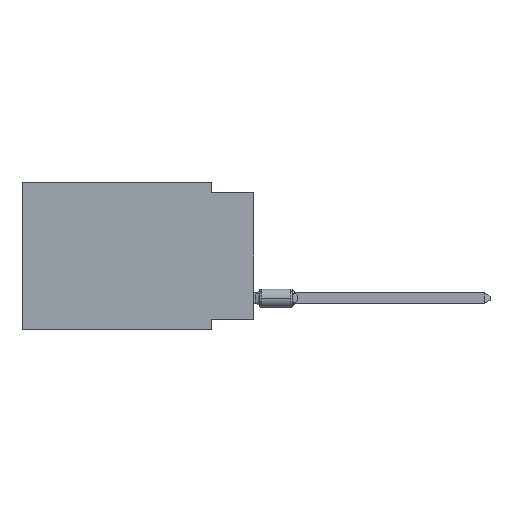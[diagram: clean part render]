
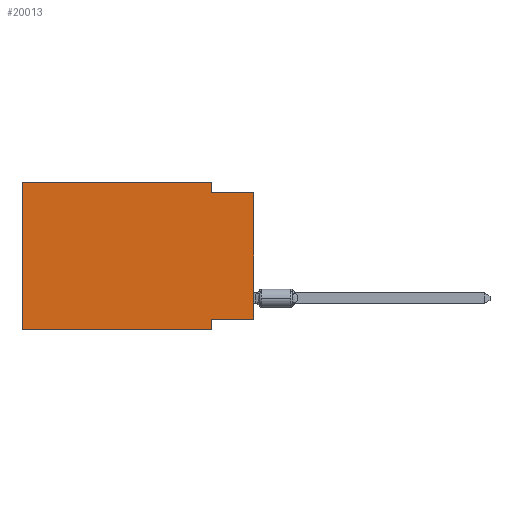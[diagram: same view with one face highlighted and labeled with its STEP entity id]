
A CAD part, left-side view. The second image highlights one B-rep face of the part: STEP entity #20013.
In plain terms, the highlighted planar face has unit normal (-1, 0, 0).
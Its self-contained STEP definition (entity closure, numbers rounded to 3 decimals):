
#96 = CARTESIAN_POINT ( 'NONE',  ( 0., 13.97, -8.89 ) ) ;
#192 = CARTESIAN_POINT ( 'NONE',  ( 0., 2.54, -8.89 ) ) ;
#899 = CARTESIAN_POINT ( 'NONE',  ( 0., 0., 0. ) ) ;
#1477 = DIRECTION ( 'NONE',  ( 0., 0., 1. ) ) ;
#1546 = DIRECTION ( 'NONE',  ( 0., -1., 0. ) ) ;
#1777 = ORIENTED_EDGE ( 'NONE', *, *, #7221, .F. ) ;
#2259 = VERTEX_POINT ( 'NONE', #11842 ) ;
#2874 = VECTOR ( 'NONE', #1546, 1000. ) ;
#2972 = PLANE ( 'NONE',  #17500 ) ;
#3095 = FACE_OUTER_BOUND ( 'NONE', #8683, .T. ) ;
#3350 = CARTESIAN_POINT ( 'NONE',  ( 0., 2.54, -8.255 ) ) ;
#3458 = EDGE_CURVE ( 'NONE', #14503, #10367, #22338, .T. ) ;
#3532 = CARTESIAN_POINT ( 'NONE',  ( 0., 13.97, 0. ) ) ;
#3950 = ORIENTED_EDGE ( 'NONE', *, *, #3458, .F. ) ;
#4339 = DIRECTION ( 'NONE',  ( 0., 0., -1. ) ) ;
#4348 = CARTESIAN_POINT ( 'NONE',  ( 0., 2.54, 0. ) ) ;
#4909 = DIRECTION ( 'NONE',  ( 1., 0., 0. ) ) ;
#5373 = ORIENTED_EDGE ( 'NONE', *, *, #11270, .T. ) ;
#5618 = EDGE_CURVE ( 'NONE', #17515, #2259, #21435, .T. ) ;
#5721 = ORIENTED_EDGE ( 'NONE', *, *, #22646, .F. ) ;
#5803 = CARTESIAN_POINT ( 'NONE',  ( 0., 2.54, 0. ) ) ;
#6016 = VECTOR ( 'NONE', #11324, 1000. ) ;
#6582 = DIRECTION ( 'NONE',  ( 0., 0., 1. ) ) ;
#6608 = VERTEX_POINT ( 'NONE', #96 ) ;
#6885 = VERTEX_POINT ( 'NONE', #3350 ) ;
#7116 = CARTESIAN_POINT ( 'NONE',  ( 0., 0., -0.635 ) ) ;
#7147 = DIRECTION ( 'NONE',  ( 0., -1., 0. ) ) ;
#7221 = EDGE_CURVE ( 'NONE', #6608, #21553, #20195, .T. ) ;
#7418 = CARTESIAN_POINT ( 'NONE',  ( 0., 13.97, -8.89 ) ) ;
#7873 = VECTOR ( 'NONE', #16521, 1000. ) ;
#8683 = EDGE_LOOP ( 'NONE', ( #16354, #18234, #3950, #23668, #1777, #5373, #22352, #5721 ) ) ;
#8732 = CARTESIAN_POINT ( 'NONE',  ( 0., 2.54, -0.635 ) ) ;
#9247 = VERTEX_POINT ( 'NONE', #23162 ) ;
#9518 = VECTOR ( 'NONE', #21668, 1000. ) ;
#10367 = VERTEX_POINT ( 'NONE', #8732 ) ;
#10372 = EDGE_CURVE ( 'NONE', #21553, #14503, #19822, .T. ) ;
#10519 = LINE ( 'NONE', #7116, #2874 ) ;
#10752 = EDGE_CURVE ( 'NONE', #10367, #2259, #10519, .T. ) ;
#11270 = EDGE_CURVE ( 'NONE', #6608, #9247, #12736, .T. ) ;
#11324 = DIRECTION ( 'NONE',  ( 0., 1., 0. ) ) ;
#11842 = CARTESIAN_POINT ( 'NONE',  ( 0., 0., -0.635 ) ) ;
#12736 = LINE ( 'NONE', #7418, #9518 ) ;
#13602 = CARTESIAN_POINT ( 'NONE',  ( 0., 13.97, 0. ) ) ;
#14503 = VERTEX_POINT ( 'NONE', #4348 ) ;
#14629 = CARTESIAN_POINT ( 'NONE',  ( 0., 13.97, 0. ) ) ;
#15099 = VECTOR ( 'NONE', #6582, 1000. ) ;
#15466 = VECTOR ( 'NONE', #1477, 1000. ) ;
#16200 = VECTOR ( 'NONE', #4339, 1000. ) ;
#16354 = ORIENTED_EDGE ( 'NONE', *, *, #5618, .T. ) ;
#16373 = VECTOR ( 'NONE', #7147, 1000. ) ;
#16463 = CARTESIAN_POINT ( 'NONE',  ( 0., 0., -8.255 ) ) ;
#16521 = DIRECTION ( 'NONE',  ( 0., 0., -1. ) ) ;
#17500 = AXIS2_PLACEMENT_3D ( 'NONE', #17831, #4909, #19392 ) ;
#17515 = VERTEX_POINT ( 'NONE', #16463 ) ;
#17831 = CARTESIAN_POINT ( 'NONE',  ( 0., 13.97, 0. ) ) ;
#18234 = ORIENTED_EDGE ( 'NONE', *, *, #10752, .F. ) ;
#18454 = EDGE_CURVE ( 'NONE', #6885, #9247, #22298, .T. ) ;
#18543 = LINE ( 'NONE', #22650, #6016 ) ;
#19392 = DIRECTION ( 'NONE',  ( 0., 0., -1. ) ) ;
#19822 = LINE ( 'NONE', #14629, #16373 ) ;
#20013 = ADVANCED_FACE ( 'NONE', ( #3095 ), #2972, .F. ) ;
#20195 = LINE ( 'NONE', #3532, #15466 ) ;
#21435 = LINE ( 'NONE', #899, #15099 ) ;
#21553 = VERTEX_POINT ( 'NONE', #13602 ) ;
#21668 = DIRECTION ( 'NONE',  ( 0., -1., 0. ) ) ;
#22298 = LINE ( 'NONE', #192, #7873 ) ;
#22338 = LINE ( 'NONE', #5803, #16200 ) ;
#22352 = ORIENTED_EDGE ( 'NONE', *, *, #18454, .F. ) ;
#22646 = EDGE_CURVE ( 'NONE', #17515, #6885, #18543, .T. ) ;
#22650 = CARTESIAN_POINT ( 'NONE',  ( 0., 0., -8.255 ) ) ;
#23162 = CARTESIAN_POINT ( 'NONE',  ( 0., 2.54, -8.89 ) ) ;
#23668 = ORIENTED_EDGE ( 'NONE', *, *, #10372, .F. ) ;
